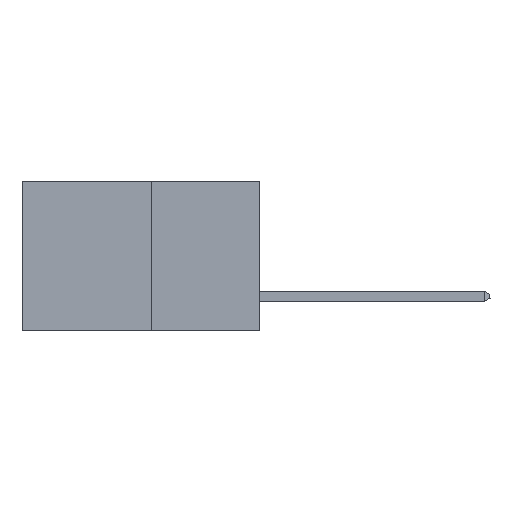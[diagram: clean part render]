
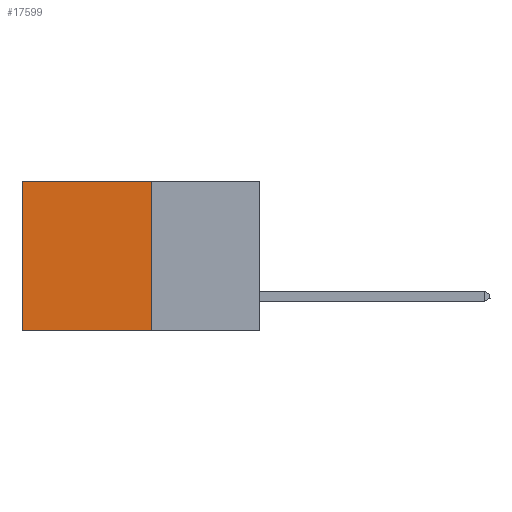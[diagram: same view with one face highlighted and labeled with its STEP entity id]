
A CAD part, left-side view. The second image highlights one B-rep face of the part: STEP entity #17599.
In plain terms, the highlighted planar face has unit normal (-1, 0, 0).
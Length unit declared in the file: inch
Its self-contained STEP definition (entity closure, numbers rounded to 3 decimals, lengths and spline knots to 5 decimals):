
#268 = EDGE_LOOP ( 'NONE', ( #10242, #13688, #2786, #17285 ) ) ;
#843 = PLANE ( 'NONE',  #4539 ) ;
#2219 = CARTESIAN_POINT ( 'NONE',  ( 0.277, 0.27, 0. ) ) ;
#2245 = VECTOR ( 'NONE', #2334, 39.37008 ) ;
#2334 = DIRECTION ( 'NONE',  ( 0., 0., -1. ) ) ;
#2764 = LINE ( 'NONE', #10296, #2245 ) ;
#2786 = ORIENTED_EDGE ( 'NONE', *, *, #8939, .F. ) ;
#3530 = CARTESIAN_POINT ( 'NONE',  ( 0.277, 0.59, -0.37 ) ) ;
#3994 = VECTOR ( 'NONE', #5070, 39.37008 ) ;
#4475 = LINE ( 'NONE', #3530, #3994 ) ;
#4539 = AXIS2_PLACEMENT_3D ( 'NONE', #12030, #16646, #7298 ) ;
#4719 = LINE ( 'NONE', #6090, #8519 ) ;
#4887 = VERTEX_POINT ( 'NONE', #12880 ) ;
#5070 = DIRECTION ( 'NONE',  ( 0., 0., -1. ) ) ;
#5214 = DIRECTION ( 'NONE',  ( 0., 1., 0. ) ) ;
#6090 = CARTESIAN_POINT ( 'NONE',  ( 0.277, 0.27, -0.37 ) ) ;
#7262 = VECTOR ( 'NONE', #5214, 39.37008 ) ;
#7298 = DIRECTION ( 'NONE',  ( 0., 0., -1. ) ) ;
#8519 = VECTOR ( 'NONE', #18587, 39.37008 ) ;
#8939 = EDGE_CURVE ( 'NONE', #15985, #11320, #2764, .T. ) ;
#10242 = ORIENTED_EDGE ( 'NONE', *, *, #17124, .T. ) ;
#10296 = CARTESIAN_POINT ( 'NONE',  ( 0.277, 0.27, -0.37 ) ) ;
#10974 = FACE_OUTER_BOUND ( 'NONE', #268, .T. ) ;
#11320 = VERTEX_POINT ( 'NONE', #14465 ) ;
#12030 = CARTESIAN_POINT ( 'NONE',  ( 0.277, 0.27, -0.37 ) ) ;
#12880 = CARTESIAN_POINT ( 'NONE',  ( 0.277, 0.59, -0.37 ) ) ;
#13688 = ORIENTED_EDGE ( 'NONE', *, *, #16866, .F. ) ;
#14465 = CARTESIAN_POINT ( 'NONE',  ( 0.277, 0.27, -0.37 ) ) ;
#15689 = CARTESIAN_POINT ( 'NONE',  ( 0.277, 0.59, 0. ) ) ;
#15985 = VERTEX_POINT ( 'NONE', #2219 ) ;
#16247 = CARTESIAN_POINT ( 'NONE',  ( 0.277, 0.27, 0. ) ) ;
#16305 = VERTEX_POINT ( 'NONE', #15689 ) ;
#16646 = DIRECTION ( 'NONE',  ( 1., 0., 0. ) ) ;
#16866 = EDGE_CURVE ( 'NONE', #11320, #4887, #4719, .T. ) ;
#17124 = EDGE_CURVE ( 'NONE', #16305, #4887, #4475, .T. ) ;
#17185 = EDGE_CURVE ( 'NONE', #15985, #16305, #19131, .T. ) ;
#17285 = ORIENTED_EDGE ( 'NONE', *, *, #17185, .T. ) ;
#17599 = ADVANCED_FACE ( 'NONE', ( #10974 ), #843, .F. ) ;
#18587 = DIRECTION ( 'NONE',  ( 0., 1., 0. ) ) ;
#19131 = LINE ( 'NONE', #16247, #7262 ) ;
